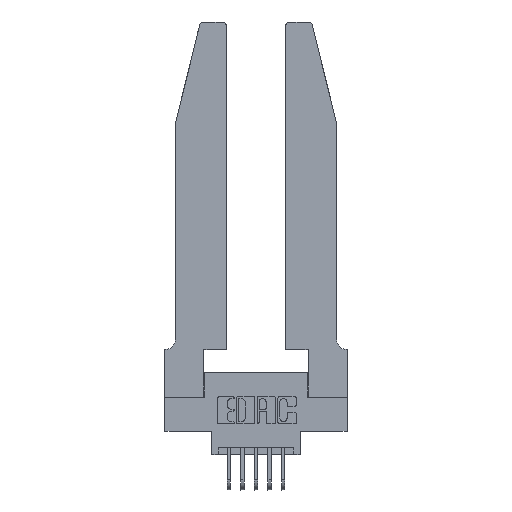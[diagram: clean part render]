
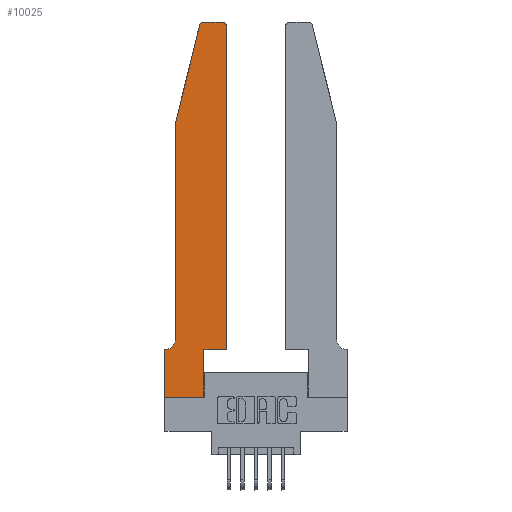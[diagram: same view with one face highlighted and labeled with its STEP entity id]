
A CAD part, top view. The second image highlights one B-rep face of the part: STEP entity #10025.
In plain terms, the highlighted planar face has unit normal (0, 0, 1).
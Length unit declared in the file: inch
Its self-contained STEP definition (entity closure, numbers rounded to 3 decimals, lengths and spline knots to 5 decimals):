
#145 = CARTESIAN_POINT ( 'NONE',  ( 0.2605, 2.75, 0.37 ) ) ;
#204 = VERTEX_POINT ( 'NONE', #12709 ) ;
#376 = DIRECTION ( 'NONE',  ( 0., 1., 0. ) ) ;
#808 = EDGE_CURVE ( 'NONE', #204, #10520, #4054, .T. ) ;
#881 = VECTOR ( 'NONE', #9287, 39.37008 ) ;
#938 = CARTESIAN_POINT ( 'NONE',  ( 0.0755, 0.35, 0.37 ) ) ;
#989 = VERTEX_POINT ( 'NONE', #15439 ) ;
#1092 = VERTEX_POINT ( 'NONE', #12151 ) ;
#1695 = PLANE ( 'NONE',  #5483 ) ;
#2446 = ORIENTED_EDGE ( 'NONE', *, *, #8269, .T. ) ;
#2514 = DIRECTION ( 'NONE',  ( -0.239, -0.971, 0. ) ) ;
#2521 = EDGE_CURVE ( 'NONE', #10520, #3640, #12024, .T. ) ;
#3041 = LINE ( 'NONE', #12158, #10682 ) ;
#3263 = ORIENTED_EDGE ( 'NONE', *, *, #8599, .T. ) ;
#3279 = CARTESIAN_POINT ( 'NONE',  ( 0., 0., 0.37 ) ) ;
#3640 = VERTEX_POINT ( 'NONE', #10858 ) ;
#3682 = VECTOR ( 'NONE', #10791, 39.37008 ) ;
#3850 = LINE ( 'NONE', #4661, #11654 ) ;
#3866 = LINE ( 'NONE', #145, #3682 ) ;
#3904 = VERTEX_POINT ( 'NONE', #11187 ) ;
#4010 = VECTOR ( 'NONE', #7932, 39.37008 ) ;
#4054 = LINE ( 'NONE', #938, #881 ) ;
#4349 = CARTESIAN_POINT ( 'NONE',  ( 0.284, 2.72, 0.37 ) ) ;
#4360 = ORIENTED_EDGE ( 'NONE', *, *, #12774, .T. ) ;
#4403 = CARTESIAN_POINT ( 'NONE',  ( 0.4505, 0.35, 0.37 ) ) ;
#4510 = ORIENTED_EDGE ( 'NONE', *, *, #2521, .T. ) ;
#4661 = CARTESIAN_POINT ( 'NONE',  ( 0.4505, 0.35, 0.37 ) ) ;
#4744 = CARTESIAN_POINT ( 'NONE',  ( 0.0755, 0.42, 0.37 ) ) ;
#4824 = LINE ( 'NONE', #4403, #10019 ) ;
#5088 = CARTESIAN_POINT ( 'NONE',  ( 0.2865, 0.35, 0.37 ) ) ;
#5328 = CARTESIAN_POINT ( 'NONE',  ( 0., 0.35, 0.37 ) ) ;
#5386 = CIRCLE ( 'NONE', #11534, 0.03 ) ;
#5437 = DIRECTION ( 'NONE',  ( 1., 0., 0. ) ) ;
#5483 = AXIS2_PLACEMENT_3D ( 'NONE', #5328, #13656, #8893 ) ;
#5583 = ORIENTED_EDGE ( 'NONE', *, *, #13491, .T. ) ;
#5615 = VERTEX_POINT ( 'NONE', #9401 ) ;
#6317 = DIRECTION ( 'NONE',  ( 0., -1., 0. ) ) ;
#6376 = CIRCLE ( 'NONE', #11786, 0.03 ) ;
#6456 = VERTEX_POINT ( 'NONE', #9613 ) ;
#6940 = CARTESIAN_POINT ( 'NONE',  ( 0.0055, 0.42, 0.37 ) ) ;
#7023 = CARTESIAN_POINT ( 'NONE',  ( 0.2865, 0., 0.37 ) ) ;
#7218 = FACE_OUTER_BOUND ( 'NONE', #7366, .T. ) ;
#7366 = EDGE_LOOP ( 'NONE', ( #11854, #13495, #11715, #14700, #5583, #15183, #4510, #4360, #2446, #3263, #11724, #13360 ) ) ;
#7695 = EDGE_CURVE ( 'NONE', #1092, #989, #5386, .T. ) ;
#7930 = VERTEX_POINT ( 'NONE', #7023 ) ;
#7932 = DIRECTION ( 'NONE',  ( 0., -1., 0. ) ) ;
#8236 = DIRECTION ( 'NONE',  ( 0., 0., 1. ) ) ;
#8269 = EDGE_CURVE ( 'NONE', #7930, #6456, #12102, .T. ) ;
#8477 = DIRECTION ( 'NONE',  ( 0., 1., 0. ) ) ;
#8516 = CARTESIAN_POINT ( 'NONE',  ( 0.4205, 2.75, 0.37 ) ) ;
#8599 = EDGE_CURVE ( 'NONE', #6456, #3904, #4824, .T. ) ;
#8893 = DIRECTION ( 'NONE',  ( 1., 0., 0. ) ) ;
#9133 = DIRECTION ( 'NONE',  ( 1., 0., 0. ) ) ;
#9158 = EDGE_CURVE ( 'NONE', #14262, #1092, #3866, .T. ) ;
#9163 = VECTOR ( 'NONE', #12930, 39.37008 ) ;
#9287 = DIRECTION ( 'NONE',  ( -1., 0., 0. ) ) ;
#9353 = DIRECTION ( 'NONE',  ( 1., 0., 0. ) ) ;
#9401 = CARTESIAN_POINT ( 'NONE',  ( 0.0755, 2., 0.37 ) ) ;
#9613 = CARTESIAN_POINT ( 'NONE',  ( 0.2865, 0.35, 0.37 ) ) ;
#9624 = LINE ( 'NONE', #13551, #12231 ) ;
#9991 = EDGE_CURVE ( 'NONE', #5615, #11174, #9624, .T. ) ;
#10019 = VECTOR ( 'NONE', #5437, 39.37008 ) ;
#10025 = ADVANCED_FACE ( 'NONE', ( #7218 ), #1695, .T. ) ;
#10520 = VERTEX_POINT ( 'NONE', #14467 ) ;
#10682 = VECTOR ( 'NONE', #2514, 39.37008 ) ;
#10748 = CIRCLE ( 'NONE', #11002, 0.07 ) ;
#10791 = DIRECTION ( 'NONE',  ( -1., 0., 0. ) ) ;
#10858 = CARTESIAN_POINT ( 'NONE',  ( 0., 0., 0.37 ) ) ;
#11002 = AXIS2_PLACEMENT_3D ( 'NONE', #6940, #14151, #12900 ) ;
#11174 = VERTEX_POINT ( 'NONE', #4744 ) ;
#11187 = CARTESIAN_POINT ( 'NONE',  ( 0.4505, 0.35, 0.37 ) ) ;
#11290 = VERTEX_POINT ( 'NONE', #13149 ) ;
#11511 = EDGE_CURVE ( 'NONE', #11290, #14262, #6376, .T. ) ;
#11534 = AXIS2_PLACEMENT_3D ( 'NONE', #4349, #12596, #9133 ) ;
#11584 = LINE ( 'NONE', #3279, #9163 ) ;
#11654 = VECTOR ( 'NONE', #8477, 39.37008 ) ;
#11715 = ORIENTED_EDGE ( 'NONE', *, *, #15376, .T. ) ;
#11724 = ORIENTED_EDGE ( 'NONE', *, *, #13705, .T. ) ;
#11786 = AXIS2_PLACEMENT_3D ( 'NONE', #13078, #8236, #9353 ) ;
#11854 = ORIENTED_EDGE ( 'NONE', *, *, #9158, .T. ) ;
#12024 = LINE ( 'NONE', #12626, #4010 ) ;
#12102 = LINE ( 'NONE', #5088, #15455 ) ;
#12151 = CARTESIAN_POINT ( 'NONE',  ( 0.284, 2.75, 0.37 ) ) ;
#12158 = CARTESIAN_POINT ( 'NONE',  ( 0.0755, 2., 0.37 ) ) ;
#12231 = VECTOR ( 'NONE', #6317, 39.37008 ) ;
#12596 = DIRECTION ( 'NONE',  ( 0., 0., 1. ) ) ;
#12626 = CARTESIAN_POINT ( 'NONE',  ( 0., 0., 0.37 ) ) ;
#12709 = CARTESIAN_POINT ( 'NONE',  ( 0.0055, 0.35, 0.37 ) ) ;
#12774 = EDGE_CURVE ( 'NONE', #3640, #7930, #11584, .T. ) ;
#12900 = DIRECTION ( 'NONE',  ( -1., 0., 0. ) ) ;
#12930 = DIRECTION ( 'NONE',  ( 1., 0., 0. ) ) ;
#13078 = CARTESIAN_POINT ( 'NONE',  ( 0.4205, 2.72, 0.37 ) ) ;
#13149 = CARTESIAN_POINT ( 'NONE',  ( 0.4505, 2.72, 0.37 ) ) ;
#13360 = ORIENTED_EDGE ( 'NONE', *, *, #11511, .T. ) ;
#13491 = EDGE_CURVE ( 'NONE', #11174, #204, #10748, .T. ) ;
#13495 = ORIENTED_EDGE ( 'NONE', *, *, #7695, .T. ) ;
#13551 = CARTESIAN_POINT ( 'NONE',  ( 0.0755, 2., 0.37 ) ) ;
#13656 = DIRECTION ( 'NONE',  ( 0., 0., 1. ) ) ;
#13705 = EDGE_CURVE ( 'NONE', #3904, #11290, #3850, .T. ) ;
#14151 = DIRECTION ( 'NONE',  ( 0., 0., -1. ) ) ;
#14262 = VERTEX_POINT ( 'NONE', #8516 ) ;
#14467 = CARTESIAN_POINT ( 'NONE',  ( 0., 0.35, 0.37 ) ) ;
#14700 = ORIENTED_EDGE ( 'NONE', *, *, #9991, .T. ) ;
#15183 = ORIENTED_EDGE ( 'NONE', *, *, #808, .T. ) ;
#15376 = EDGE_CURVE ( 'NONE', #989, #5615, #3041, .T. ) ;
#15439 = CARTESIAN_POINT ( 'NONE',  ( 0.25487, 2.72718, 0.37 ) ) ;
#15455 = VECTOR ( 'NONE', #376, 39.37008 ) ;
